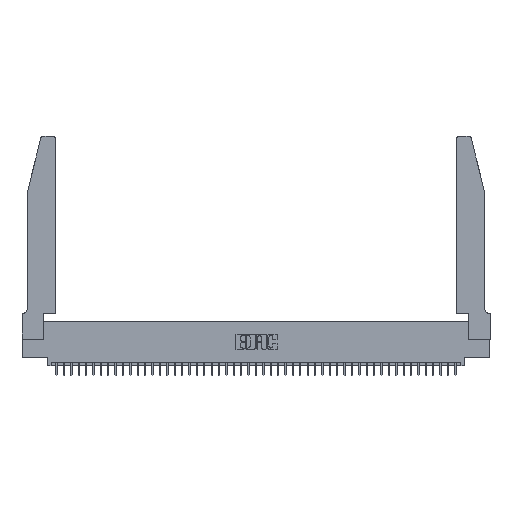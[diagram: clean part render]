
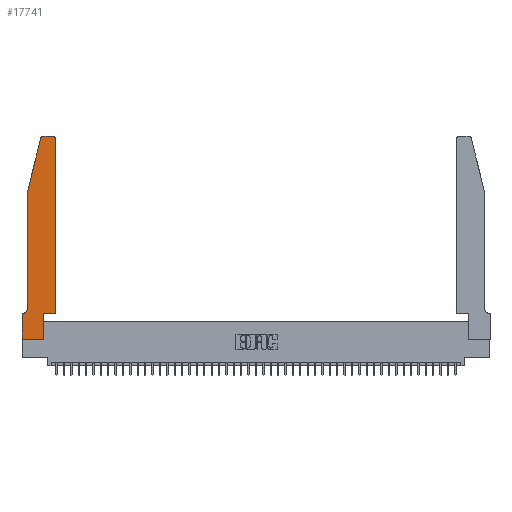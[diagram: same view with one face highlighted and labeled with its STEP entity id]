
A CAD part, top view. The second image highlights one B-rep face of the part: STEP entity #17741.
In plain terms, the highlighted planar face has unit normal (0, 0, 1).
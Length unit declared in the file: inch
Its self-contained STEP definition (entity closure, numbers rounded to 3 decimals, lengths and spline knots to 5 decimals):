
#189 = ORIENTED_EDGE ( 'NONE', *, *, #22832, .T. ) ;
#400 = ORIENTED_EDGE ( 'NONE', *, *, #28873, .T. ) ;
#463 = ORIENTED_EDGE ( 'NONE', *, *, #661, .T. ) ;
#661 = EDGE_CURVE ( 'NONE', #11904, #45919, #9667, .T. ) ;
#684 = EDGE_CURVE ( 'NONE', #27415, #40610, #30560, .T. ) ;
#845 = CARTESIAN_POINT ( 'NONE',  ( 0., 0.35, 0.37 ) ) ;
#866 = VERTEX_POINT ( 'NONE', #9125 ) ;
#1107 = ORIENTED_EDGE ( 'NONE', *, *, #684, .T. ) ;
#1214 = DIRECTION ( 'NONE',  ( 0., 0., 1. ) ) ;
#1310 = DIRECTION ( 'NONE',  ( 0., 0., 1. ) ) ;
#1394 = VERTEX_POINT ( 'NONE', #23826 ) ;
#2284 = ORIENTED_EDGE ( 'NONE', *, *, #8505, .T. ) ;
#2621 = CARTESIAN_POINT ( 'NONE',  ( 0.0755, 0.35, 0.37 ) ) ;
#3653 = CIRCLE ( 'NONE', #19392, 0.03 ) ;
#4761 = VECTOR ( 'NONE', #16959, 39.37008 ) ;
#6330 = ORIENTED_EDGE ( 'NONE', *, *, #11290, .T. ) ;
#6358 = DIRECTION ( 'NONE',  ( 0., 1., 0. ) ) ;
#6501 = VERTEX_POINT ( 'NONE', #11049 ) ;
#6884 = CARTESIAN_POINT ( 'NONE',  ( 0., 0.35, 0.37 ) ) ;
#7568 = CARTESIAN_POINT ( 'NONE',  ( 0.284, 2.75, 0.37 ) ) ;
#7761 = ORIENTED_EDGE ( 'NONE', *, *, #9486, .T. ) ;
#7763 = LINE ( 'NONE', #18073, #37060 ) ;
#8136 = DIRECTION ( 'NONE',  ( 1., 0., 0. ) ) ;
#8148 = VECTOR ( 'NONE', #41579, 39.37008 ) ;
#8403 = AXIS2_PLACEMENT_3D ( 'NONE', #42232, #28378, #17088 ) ;
#8505 = EDGE_CURVE ( 'NONE', #1394, #27027, #9112, .T. ) ;
#8685 = DIRECTION ( 'NONE',  ( 0., 0., -1. ) ) ;
#8962 = DIRECTION ( 'NONE',  ( 1., 0., 0. ) ) ;
#9112 = LINE ( 'NONE', #19657, #38736 ) ;
#9125 = CARTESIAN_POINT ( 'NONE',  ( 0.2865, 0.35, 0.37 ) ) ;
#9486 = EDGE_CURVE ( 'NONE', #35525, #13487, #41632, .T. ) ;
#9667 = LINE ( 'NONE', #23969, #34087 ) ;
#9731 = VECTOR ( 'NONE', #33379, 39.37008 ) ;
#9733 = CARTESIAN_POINT ( 'NONE',  ( 0.0755, 0.42, 0.37 ) ) ;
#11049 = CARTESIAN_POINT ( 'NONE',  ( 0., 0., 0.37 ) ) ;
#11129 = EDGE_CURVE ( 'NONE', #27027, #15335, #3653, .T. ) ;
#11290 = EDGE_CURVE ( 'NONE', #6501, #16616, #19979, .T. ) ;
#11515 = LINE ( 'NONE', #25381, #9731 ) ;
#11531 = CARTESIAN_POINT ( 'NONE',  ( 0.284, 2.72, 0.37 ) ) ;
#11904 = VERTEX_POINT ( 'NONE', #40090 ) ;
#12244 = AXIS2_PLACEMENT_3D ( 'NONE', #45057, #8685, #44363 ) ;
#12897 = CIRCLE ( 'NONE', #8403, 0.03 ) ;
#13214 = CARTESIAN_POINT ( 'NONE',  ( 0.4505, 0.35, 0.37 ) ) ;
#13432 = CARTESIAN_POINT ( 'NONE',  ( 0.25487, 2.72718, 0.37 ) ) ;
#13487 = VERTEX_POINT ( 'NONE', #40272 ) ;
#15335 = VERTEX_POINT ( 'NONE', #13432 ) ;
#16616 = VERTEX_POINT ( 'NONE', #27774 ) ;
#16959 = DIRECTION ( 'NONE',  ( 0., 1., 0. ) ) ;
#17088 = DIRECTION ( 'NONE',  ( 1., 0., 0. ) ) ;
#17741 = ADVANCED_FACE ( 'NONE', ( #29722 ), #40284, .T. ) ;
#17811 = LINE ( 'NONE', #21123, #31497 ) ;
#18073 = CARTESIAN_POINT ( 'NONE',  ( 0., 0., 0.37 ) ) ;
#19392 = AXIS2_PLACEMENT_3D ( 'NONE', #11531, #1214, #8962 ) ;
#19465 = LINE ( 'NONE', #30502, #35319 ) ;
#19657 = CARTESIAN_POINT ( 'NONE',  ( 0.2605, 2.75, 0.37 ) ) ;
#19828 = VECTOR ( 'NONE', #27287, 39.37008 ) ;
#19979 = LINE ( 'NONE', #34775, #8148 ) ;
#20617 = ORIENTED_EDGE ( 'NONE', *, *, #22522, .T. ) ;
#21123 = CARTESIAN_POINT ( 'NONE',  ( 0.2865, 0.35, 0.37 ) ) ;
#21835 = DIRECTION ( 'NONE',  ( 0., -1., 0. ) ) ;
#22522 = EDGE_CURVE ( 'NONE', #866, #35525, #11515, .T. ) ;
#22832 = EDGE_CURVE ( 'NONE', #16616, #866, #17811, .T. ) ;
#23057 = ORIENTED_EDGE ( 'NONE', *, *, #11129, .T. ) ;
#23826 = CARTESIAN_POINT ( 'NONE',  ( 0.4205, 2.75, 0.37 ) ) ;
#23969 = CARTESIAN_POINT ( 'NONE',  ( 0.0755, 2., 0.37 ) ) ;
#25381 = CARTESIAN_POINT ( 'NONE',  ( 0.4505, 0.35, 0.37 ) ) ;
#25782 = EDGE_CURVE ( 'NONE', #15335, #11904, #19465, .T. ) ;
#27027 = VERTEX_POINT ( 'NONE', #7568 ) ;
#27112 = AXIS2_PLACEMENT_3D ( 'NONE', #845, #1310, #8136 ) ;
#27287 = DIRECTION ( 'NONE',  ( -1., 0., 0. ) ) ;
#27415 = VERTEX_POINT ( 'NONE', #28656 ) ;
#27455 = DIRECTION ( 'NONE',  ( -0.239, -0.971, 0. ) ) ;
#27774 = CARTESIAN_POINT ( 'NONE',  ( 0.2865, 0., 0.37 ) ) ;
#28061 = ORIENTED_EDGE ( 'NONE', *, *, #25782, .T. ) ;
#28378 = DIRECTION ( 'NONE',  ( 0., 0., 1. ) ) ;
#28656 = CARTESIAN_POINT ( 'NONE',  ( 0.0055, 0.35, 0.37 ) ) ;
#28873 = EDGE_CURVE ( 'NONE', #45919, #27415, #34753, .T. ) ;
#29722 = FACE_OUTER_BOUND ( 'NONE', #35880, .T. ) ;
#30175 = EDGE_CURVE ( 'NONE', #40610, #6501, #7763, .T. ) ;
#30502 = CARTESIAN_POINT ( 'NONE',  ( 0.0755, 2., 0.37 ) ) ;
#30560 = LINE ( 'NONE', #2621, #19828 ) ;
#31497 = VECTOR ( 'NONE', #6358, 39.37008 ) ;
#33379 = DIRECTION ( 'NONE',  ( 1., 0., 0. ) ) ;
#34087 = VECTOR ( 'NONE', #45120, 39.37008 ) ;
#34452 = ORIENTED_EDGE ( 'NONE', *, *, #30175, .T. ) ;
#34753 = CIRCLE ( 'NONE', #12244, 0.07 ) ;
#34775 = CARTESIAN_POINT ( 'NONE',  ( 0., 0., 0.37 ) ) ;
#35319 = VECTOR ( 'NONE', #27455, 39.37008 ) ;
#35525 = VERTEX_POINT ( 'NONE', #37968 ) ;
#35880 = EDGE_LOOP ( 'NONE', ( #2284, #23057, #28061, #463, #400, #1107, #34452, #6330, #189, #20617, #7761, #42660 ) ) ;
#37060 = VECTOR ( 'NONE', #21835, 39.37008 ) ;
#37509 = DIRECTION ( 'NONE',  ( -1., 0., 0. ) ) ;
#37968 = CARTESIAN_POINT ( 'NONE',  ( 0.4505, 0.35, 0.37 ) ) ;
#38736 = VECTOR ( 'NONE', #37509, 39.37008 ) ;
#40090 = CARTESIAN_POINT ( 'NONE',  ( 0.0755, 2., 0.37 ) ) ;
#40272 = CARTESIAN_POINT ( 'NONE',  ( 0.4505, 2.72, 0.37 ) ) ;
#40284 = PLANE ( 'NONE',  #27112 ) ;
#40610 = VERTEX_POINT ( 'NONE', #6884 ) ;
#41579 = DIRECTION ( 'NONE',  ( 1., 0., 0. ) ) ;
#41632 = LINE ( 'NONE', #13214, #4761 ) ;
#42232 = CARTESIAN_POINT ( 'NONE',  ( 0.4205, 2.72, 0.37 ) ) ;
#42660 = ORIENTED_EDGE ( 'NONE', *, *, #42707, .T. ) ;
#42707 = EDGE_CURVE ( 'NONE', #13487, #1394, #12897, .T. ) ;
#44363 = DIRECTION ( 'NONE',  ( -1., 0., 0. ) ) ;
#45057 = CARTESIAN_POINT ( 'NONE',  ( 0.0055, 0.42, 0.37 ) ) ;
#45120 = DIRECTION ( 'NONE',  ( 0., -1., 0. ) ) ;
#45919 = VERTEX_POINT ( 'NONE', #9733 ) ;
